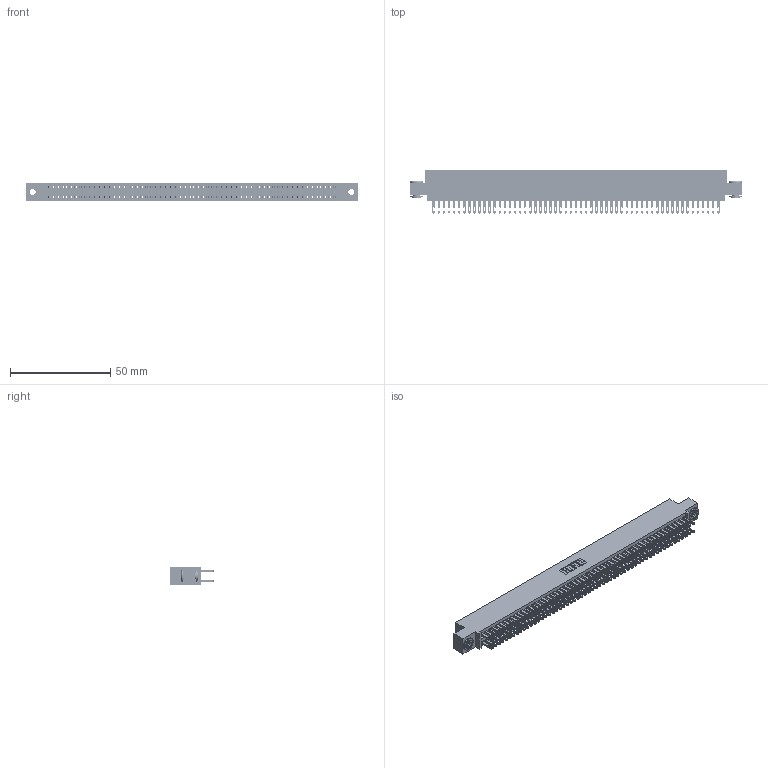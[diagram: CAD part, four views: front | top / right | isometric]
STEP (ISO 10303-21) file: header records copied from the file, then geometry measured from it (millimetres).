
FILE_DESCRIPTION (( 'STEP AP203' ), '1' );
FILE_NAME ('345-114-500-503.STEP', '2019-11-05T00:33:58', ( '' ), ( '' ), 'SwSTEP 2.0', 'SolidWorks 2016', '' );
FILE_SCHEMA (( 'CONFIG_CONTROL_DESIGN' ));
Length unit declared in the file: inch
Products named in the file (4): 345-292-001_345-293-100; 345 Part_0.110 Offset - 0.156 Dia-TH; 345-250-002_345-250-002-102; 345-114-500-503
Assembly tree (117 placements, depth 2):
  345-114-500-503
    345 Part_0.110 Offset - 0.156 Dia-TH
    345-292-001_345-293-100  x114
    345-250-002_345-250-002-102  x2
Bounding box: 165.99 x 21.51 x 9.4 mm (x, y, z)
Volume: 16558 mm3; surface area: 26226.4 mm2
Topology: 117 solids, 117 shells, 5412 faces, 16503 edges, 10998 vertices
Faces by surface type: plane 3172, cylinder 2232, cone 8
Entity records: 43416 total; most frequent: CARTESIAN_POINT 7239, ORIENTED_EDGE 7166, DIRECTION 6397, EDGE_CURVE 3583, LINE 3195, VECTOR 3195, VERTEX_POINT 2386, AXIS2_PLACEMENT_3D 1601
